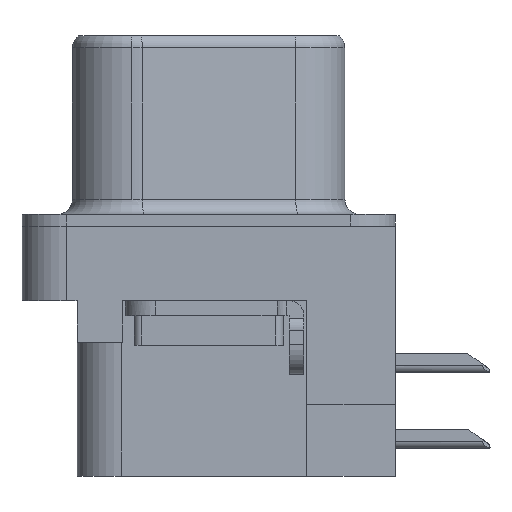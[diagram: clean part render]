
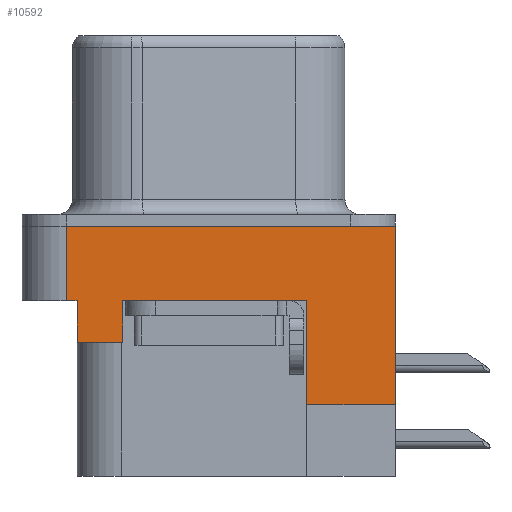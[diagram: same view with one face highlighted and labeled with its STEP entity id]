
A CAD part, left-side view. The second image highlights one B-rep face of the part: STEP entity #10592.
In plain terms, the highlighted planar face has unit normal (-1, 0, 0).
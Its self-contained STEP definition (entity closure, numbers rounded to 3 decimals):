
#154 = EDGE_CURVE ( 'NONE', #14428, #6901, #5418, .T. ) ;
#326 = ORIENTED_EDGE ( 'NONE', *, *, #1449, .F. ) ;
#418 = CARTESIAN_POINT ( 'NONE',  ( -2.935, 2.895, -3.9 ) ) ;
#455 = ORIENTED_EDGE ( 'NONE', *, *, #1363, .T. ) ;
#610 = CARTESIAN_POINT ( 'NONE',  ( -2.935, 4.775, -2.5 ) ) ;
#699 = CARTESIAN_POINT ( 'NONE',  ( -2.935, -3.295, -8.4 ) ) ;
#1117 = EDGE_CURVE ( 'NONE', #9604, #4955, #6438, .T. ) ;
#1185 = CARTESIAN_POINT ( 'NONE',  ( -2.935, -6.275, -2.5 ) ) ;
#1214 = EDGE_CURVE ( 'NONE', #14428, #9604, #10869, .T. ) ;
#1363 = EDGE_CURVE ( 'NONE', #2674, #2080, #12237, .T. ) ;
#1421 = EDGE_CURVE ( 'NONE', #3754, #9944, #14286, .T. ) ;
#1424 = EDGE_CURVE ( 'NONE', #3754, #13999, #10659, .T. ) ;
#1431 = EDGE_CURVE ( 'NONE', #14745, #13999, #4586, .T. ) ;
#1448 = EDGE_CURVE ( 'NONE', #2674, #14745, #13554, .T. ) ;
#1449 = EDGE_CURVE ( 'NONE', #6901, #2080, #16243, .T. ) ;
#1451 = EDGE_CURVE ( 'NONE', #9944, #4955, #9774, .T. ) ;
#1498 = DIRECTION ( 'NONE',  ( 0., 0., 1. ) ) ;
#2080 = VERTEX_POINT ( 'NONE', #4800 ) ;
#2524 = VECTOR ( 'NONE', #10469, 1000. ) ;
#2674 = VERTEX_POINT ( 'NONE', #13384 ) ;
#2712 = ORIENTED_EDGE ( 'NONE', *, *, #1431, .F. ) ;
#2823 = PLANE ( 'NONE',  #12165 ) ;
#2932 = VECTOR ( 'NONE', #14226, 1000. ) ;
#3270 = CARTESIAN_POINT ( 'NONE',  ( -2.935, 4.775, 0. ) ) ;
#3335 = VECTOR ( 'NONE', #6703, 1000. ) ;
#3413 = CARTESIAN_POINT ( 'NONE',  ( -2.935, -6.275, -2.5 ) ) ;
#3754 = VERTEX_POINT ( 'NONE', #12135 ) ;
#3808 = ORIENTED_EDGE ( 'NONE', *, *, #154, .F. ) ;
#4016 = CARTESIAN_POINT ( 'NONE',  ( -2.935, 2.895, -2.5 ) ) ;
#4137 = CARTESIAN_POINT ( 'NONE',  ( -2.935, -6.275, -2.5 ) ) ;
#4586 = LINE ( 'NONE', #15065, #10224 ) ;
#4800 = CARTESIAN_POINT ( 'NONE',  ( -2.935, 4.425, -2.5 ) ) ;
#4955 = VERTEX_POINT ( 'NONE', #6458 ) ;
#5418 = LINE ( 'NONE', #13524, #8779 ) ;
#5485 = DIRECTION ( 'NONE',  ( -1., 0., 0. ) ) ;
#6393 = CARTESIAN_POINT ( 'NONE',  ( -2.935, -6.275, 0. ) ) ;
#6438 = LINE ( 'NONE', #10450, #2524 ) ;
#6458 = CARTESIAN_POINT ( 'NONE',  ( -2.935, -3.295, -2.5 ) ) ;
#6703 = DIRECTION ( 'NONE',  ( 0., 0., 1. ) ) ;
#6901 = VERTEX_POINT ( 'NONE', #10626 ) ;
#7181 = VECTOR ( 'NONE', #16054, 1000. ) ;
#7849 = ORIENTED_EDGE ( 'NONE', *, *, #1421, .F. ) ;
#8779 = VECTOR ( 'NONE', #13556, 1000. ) ;
#9604 = VERTEX_POINT ( 'NONE', #4016 ) ;
#9774 = LINE ( 'NONE', #699, #2932 ) ;
#9944 = VERTEX_POINT ( 'NONE', #13775 ) ;
#10224 = VECTOR ( 'NONE', #14716, 1000. ) ;
#10450 = CARTESIAN_POINT ( 'NONE',  ( -2.935, -6.275, -2.5 ) ) ;
#10469 = DIRECTION ( 'NONE',  ( 0., -1., 0. ) ) ;
#10592 = ADVANCED_FACE ( 'NONE', ( #15918 ), #2823, .T. ) ;
#10626 = CARTESIAN_POINT ( 'NONE',  ( -2.935, 4.425, -3.9 ) ) ;
#10659 = LINE ( 'NONE', #1185, #7181 ) ;
#10869 = LINE ( 'NONE', #13748, #14111 ) ;
#11464 = VECTOR ( 'NONE', #16136, 1000. ) ;
#11608 = ORIENTED_EDGE ( 'NONE', *, *, #1117, .T. ) ;
#11631 = EDGE_LOOP ( 'NONE', ( #7849, #14333, #2712, #13129, #455, #326, #3808, #11832, #11608, #15081 ) ) ;
#11832 = ORIENTED_EDGE ( 'NONE', *, *, #1214, .T. ) ;
#12135 = CARTESIAN_POINT ( 'NONE',  ( -2.935, -6.275, -6. ) ) ;
#12165 = AXIS2_PLACEMENT_3D ( 'NONE', #4137, #5485, #14296 ) ;
#12237 = LINE ( 'NONE', #3413, #11464 ) ;
#12325 = CARTESIAN_POINT ( 'NONE',  ( -2.935, -6.495, -6. ) ) ;
#13129 = ORIENTED_EDGE ( 'NONE', *, *, #1448, .F. ) ;
#13172 = VECTOR ( 'NONE', #1498, 1000. ) ;
#13384 = CARTESIAN_POINT ( 'NONE',  ( -2.935, 4.775, -2.5 ) ) ;
#13524 = CARTESIAN_POINT ( 'NONE',  ( -2.935, 4.425, -3.9 ) ) ;
#13554 = LINE ( 'NONE', #610, #13172 ) ;
#13556 = DIRECTION ( 'NONE',  ( 0., 1., 0. ) ) ;
#13577 = DIRECTION ( 'NONE',  ( 0., 0., 1. ) ) ;
#13748 = CARTESIAN_POINT ( 'NONE',  ( -2.935, 2.895, -3.9 ) ) ;
#13775 = CARTESIAN_POINT ( 'NONE',  ( -2.935, -3.295, -6. ) ) ;
#13932 = VECTOR ( 'NONE', #16276, 1000. ) ;
#13999 = VERTEX_POINT ( 'NONE', #6393 ) ;
#14111 = VECTOR ( 'NONE', #13577, 1000. ) ;
#14226 = DIRECTION ( 'NONE',  ( 0., 0., 1. ) ) ;
#14286 = LINE ( 'NONE', #12325, #13932 ) ;
#14296 = DIRECTION ( 'NONE',  ( 0., 0., 1. ) ) ;
#14333 = ORIENTED_EDGE ( 'NONE', *, *, #1424, .T. ) ;
#14428 = VERTEX_POINT ( 'NONE', #418 ) ;
#14657 = CARTESIAN_POINT ( 'NONE',  ( -2.935, 4.425, -3.9 ) ) ;
#14716 = DIRECTION ( 'NONE',  ( 0., -1., 0. ) ) ;
#14745 = VERTEX_POINT ( 'NONE', #3270 ) ;
#15065 = CARTESIAN_POINT ( 'NONE',  ( -2.935, -6.275, 0. ) ) ;
#15081 = ORIENTED_EDGE ( 'NONE', *, *, #1451, .F. ) ;
#15918 = FACE_OUTER_BOUND ( 'NONE', #11631, .T. ) ;
#16054 = DIRECTION ( 'NONE',  ( 0., 0., 1. ) ) ;
#16136 = DIRECTION ( 'NONE',  ( 0., -1., 0. ) ) ;
#16243 = LINE ( 'NONE', #14657, #3335 ) ;
#16276 = DIRECTION ( 'NONE',  ( 0., 1., 0. ) ) ;
